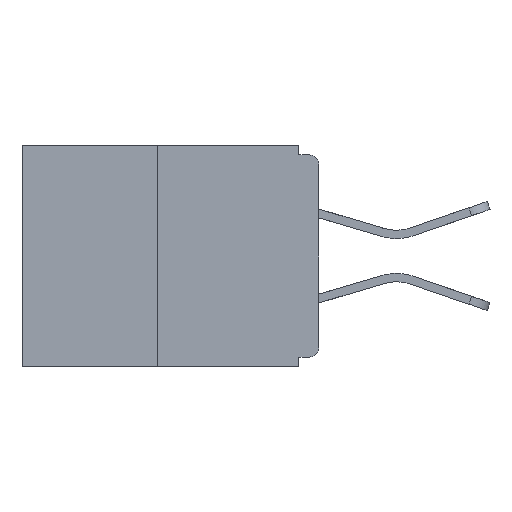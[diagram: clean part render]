
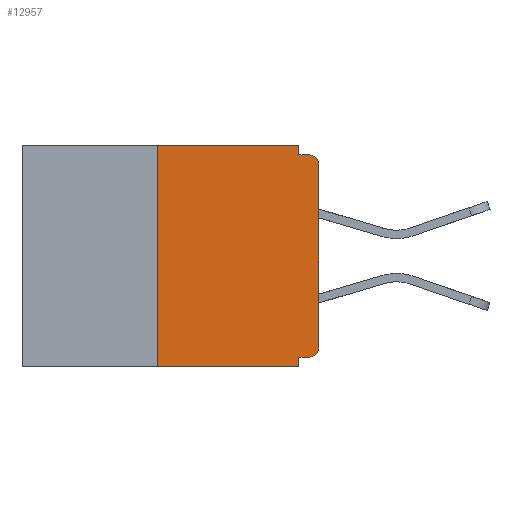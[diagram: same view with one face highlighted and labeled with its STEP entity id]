
A CAD part, left-side view. The second image highlights one B-rep face of the part: STEP entity #12957.
In plain terms, the highlighted planar face has unit normal (-1, 0, 0).
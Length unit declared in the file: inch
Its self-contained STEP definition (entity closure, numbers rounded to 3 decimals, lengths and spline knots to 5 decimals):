
#214 = EDGE_CURVE ( 'NONE', #8238, #11635, #19180, .T. ) ;
#269 = ORIENTED_EDGE ( 'NONE', *, *, #11885, .T. ) ;
#370 = DIRECTION ( 'NONE',  ( 0., 0., -1. ) ) ;
#882 = DIRECTION ( 'NONE',  ( 0., -1., 0. ) ) ;
#902 = CARTESIAN_POINT ( 'NONE',  ( 0., 0.25, -0.343 ) ) ;
#911 = DIRECTION ( 'NONE',  ( 0., -1., 0. ) ) ;
#965 = LINE ( 'NONE', #7311, #16723 ) ;
#974 = CIRCLE ( 'NONE', #2275, 0.015 ) ;
#1144 = EDGE_CURVE ( 'NONE', #15629, #3722, #965, .T. ) ;
#1453 = LINE ( 'NONE', #9470, #5138 ) ;
#1833 = CARTESIAN_POINT ( 'NONE',  ( 0., 0.46, -0.343 ) ) ;
#2215 = VECTOR ( 'NONE', #16475, 39.37008 ) ;
#2275 = AXIS2_PLACEMENT_3D ( 'NONE', #10351, #13669, #14914 ) ;
#2360 = VERTEX_POINT ( 'NONE', #14483 ) ;
#2719 = DIRECTION ( 'NONE',  ( 0., 0., 1. ) ) ;
#2840 = ORIENTED_EDGE ( 'NONE', *, *, #13591, .F. ) ;
#2959 = CARTESIAN_POINT ( 'NONE',  ( 0., 0.031, 0. ) ) ;
#3142 = CARTESIAN_POINT ( 'NONE',  ( 0., 0.031, -0.015 ) ) ;
#3169 = CARTESIAN_POINT ( 'NONE',  ( 0., 0., -0.313 ) ) ;
#3291 = EDGE_CURVE ( 'NONE', #7164, #3632, #1453, .T. ) ;
#3514 = CARTESIAN_POINT ( 'NONE',  ( 0., 0.46, 0. ) ) ;
#3632 = VERTEX_POINT ( 'NONE', #14100 ) ;
#3722 = VERTEX_POINT ( 'NONE', #17800 ) ;
#4543 = CARTESIAN_POINT ( 'NONE',  ( 0., 0.015, -0.015 ) ) ;
#4963 = LINE ( 'NONE', #1833, #17667 ) ;
#5070 = FACE_OUTER_BOUND ( 'NONE', #6224, .T. ) ;
#5138 = VECTOR ( 'NONE', #12493, 39.37008 ) ;
#5704 = ORIENTED_EDGE ( 'NONE', *, *, #15206, .T. ) ;
#5721 = CARTESIAN_POINT ( 'NONE',  ( 0., 0.031, 0. ) ) ;
#6224 = EDGE_LOOP ( 'NONE', ( #7696, #10390, #5704, #12651, #20500, #13042, #8668, #269, #13831, #2840 ) ) ;
#7123 = CARTESIAN_POINT ( 'NONE',  ( 0., 0.015, -0.03 ) ) ;
#7164 = VERTEX_POINT ( 'NONE', #19649 ) ;
#7226 = LINE ( 'NONE', #12224, #19237 ) ;
#7230 = CIRCLE ( 'NONE', #15526, 0.015 ) ;
#7260 = CARTESIAN_POINT ( 'NONE',  ( 0., 0., -0.015 ) ) ;
#7311 = CARTESIAN_POINT ( 'NONE',  ( 0., 0., 0. ) ) ;
#7455 = VECTOR ( 'NONE', #911, 39.37008 ) ;
#7665 = LINE ( 'NONE', #2959, #8594 ) ;
#7696 = ORIENTED_EDGE ( 'NONE', *, *, #10793, .F. ) ;
#7937 = AXIS2_PLACEMENT_3D ( 'NONE', #3514, #8616, #13176 ) ;
#8087 = DIRECTION ( 'NONE',  ( 0., -1., 0. ) ) ;
#8238 = VERTEX_POINT ( 'NONE', #3142 ) ;
#8594 = VECTOR ( 'NONE', #9205, 39.37008 ) ;
#8616 = DIRECTION ( 'NONE',  ( 1., 0., 0. ) ) ;
#8668 = ORIENTED_EDGE ( 'NONE', *, *, #1144, .T. ) ;
#9205 = DIRECTION ( 'NONE',  ( 0., 0., -1. ) ) ;
#9276 = CARTESIAN_POINT ( 'NONE',  ( 0., 0.25, 0. ) ) ;
#9470 = CARTESIAN_POINT ( 'NONE',  ( 0., 0., -0.328 ) ) ;
#10162 = LINE ( 'NONE', #19638, #2215 ) ;
#10351 = CARTESIAN_POINT ( 'NONE',  ( 0., 0.015, -0.313 ) ) ;
#10390 = ORIENTED_EDGE ( 'NONE', *, *, #17050, .F. ) ;
#10793 = EDGE_CURVE ( 'NONE', #2360, #14655, #7226, .T. ) ;
#10939 = VERTEX_POINT ( 'NONE', #11255 ) ;
#11255 = CARTESIAN_POINT ( 'NONE',  ( 0., 0.031, -0.343 ) ) ;
#11635 = VERTEX_POINT ( 'NONE', #4543 ) ;
#11885 = EDGE_CURVE ( 'NONE', #3722, #11635, #7230, .T. ) ;
#12224 = CARTESIAN_POINT ( 'NONE',  ( 0., 0.46, 0. ) ) ;
#12493 = DIRECTION ( 'NONE',  ( 0., 1., 0. ) ) ;
#12651 = ORIENTED_EDGE ( 'NONE', *, *, #17725, .F. ) ;
#12957 = ADVANCED_FACE ( 'NONE', ( #5070 ), #13282, .F. ) ;
#13042 = ORIENTED_EDGE ( 'NONE', *, *, #19485, .T. ) ;
#13176 = DIRECTION ( 'NONE',  ( 0., 0., -1. ) ) ;
#13282 = PLANE ( 'NONE',  #7937 ) ;
#13591 = EDGE_CURVE ( 'NONE', #14655, #8238, #7665, .T. ) ;
#13669 = DIRECTION ( 'NONE',  ( -1., 0., 0. ) ) ;
#13831 = ORIENTED_EDGE ( 'NONE', *, *, #214, .F. ) ;
#14100 = CARTESIAN_POINT ( 'NONE',  ( 0., 0.031, -0.328 ) ) ;
#14411 = VECTOR ( 'NONE', #2719, 39.37008 ) ;
#14483 = CARTESIAN_POINT ( 'NONE',  ( 0., 0.25, 0. ) ) ;
#14620 = DIRECTION ( 'NONE',  ( -1., 0., 0. ) ) ;
#14655 = VERTEX_POINT ( 'NONE', #5721 ) ;
#14914 = DIRECTION ( 'NONE',  ( 0., 0., -1. ) ) ;
#15206 = EDGE_CURVE ( 'NONE', #17944, #10939, #4963, .T. ) ;
#15308 = LINE ( 'NONE', #9276, #14411 ) ;
#15526 = AXIS2_PLACEMENT_3D ( 'NONE', #7123, #14620, #370 ) ;
#15629 = VERTEX_POINT ( 'NONE', #3169 ) ;
#16475 = DIRECTION ( 'NONE',  ( 0., 0., -1. ) ) ;
#16723 = VECTOR ( 'NONE', #18314, 39.37008 ) ;
#17050 = EDGE_CURVE ( 'NONE', #17944, #2360, #15308, .T. ) ;
#17667 = VECTOR ( 'NONE', #8087, 39.37008 ) ;
#17725 = EDGE_CURVE ( 'NONE', #3632, #10939, #10162, .T. ) ;
#17800 = CARTESIAN_POINT ( 'NONE',  ( 0., 0., -0.03 ) ) ;
#17944 = VERTEX_POINT ( 'NONE', #902 ) ;
#18314 = DIRECTION ( 'NONE',  ( 0., 0., 1. ) ) ;
#19180 = LINE ( 'NONE', #7260, #7455 ) ;
#19237 = VECTOR ( 'NONE', #882, 39.37008 ) ;
#19485 = EDGE_CURVE ( 'NONE', #7164, #15629, #974, .T. ) ;
#19638 = CARTESIAN_POINT ( 'NONE',  ( 0., 0.031, -0.343 ) ) ;
#19649 = CARTESIAN_POINT ( 'NONE',  ( 0., 0.015, -0.328 ) ) ;
#20500 = ORIENTED_EDGE ( 'NONE', *, *, #3291, .F. ) ;
